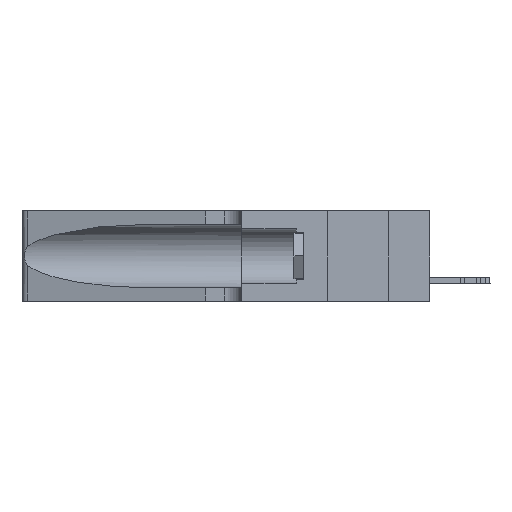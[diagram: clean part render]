
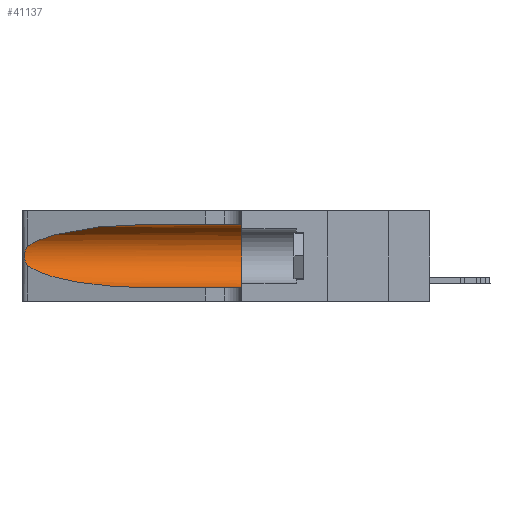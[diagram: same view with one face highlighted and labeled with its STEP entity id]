
A CAD part, left-side view. The second image highlights one B-rep face of the part: STEP entity #41137.
In plain terms, the highlighted cylindrical face has radius 3.308 mm (diameter 6.617 mm), a partial arc.
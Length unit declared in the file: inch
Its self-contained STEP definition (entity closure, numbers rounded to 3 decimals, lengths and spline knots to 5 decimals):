
#119 = CARTESIAN_POINT ( 'NONE',  ( 0.18966, 0.96281, 0.31525 ) ) ;
#580 = CARTESIAN_POINT ( 'NONE',  ( 0.26075, 1.23896, 0.178 ) ) ;
#2409 = B_SPLINE_CURVE_WITH_KNOTS ( 'NONE', 3,
 ( #41883, #7510, #21399, #31585, #34873, #38755, #18142, #580, #25042, #31433, #24588, #38159, #35306, #28150 ),
 .UNSPECIFIED., .F., .F.,
 ( 4, 2, 2, 2, 2, 2, 4 ),
 ( 0., 0.00027, 0.00053, 0.00107, 0.0016, 0.00187, 0.00214 ),
 .UNSPECIFIED. ) ;
#3069 = DIRECTION ( 'NONE',  ( 0., 0., -1. ) ) ;
#3190 = EDGE_CURVE ( 'NONE', #4982, #40101, #2409, .T. ) ;
#4982 = VERTEX_POINT ( 'NONE', #12054 ) ;
#5468 = EDGE_LOOP ( 'NONE', ( #38649, #18389, #15389, #16194, #5944, #16312 ) ) ;
#5537 = DIRECTION ( 'NONE',  ( 0., 1., 0. ) ) ;
#5944 = ORIENTED_EDGE ( 'NONE', *, *, #43632, .F. ) ;
#6344 = DIRECTION ( 'NONE',  ( 0., -1., 0. ) ) ;
#7048 = CARTESIAN_POINT ( 'NONE',  ( 0.25487, 1.22718, 0.22369 ) ) ;
#7213 = LINE ( 'NONE', #14071, #25946 ) ;
#7510 = CARTESIAN_POINT ( 'NONE',  ( 0.25555, 1.22994, 0.2215 ) ) ;
#9076 = CARTESIAN_POINT ( 'NONE',  ( 0.25487, 1.22718, 0.14631 ) ) ;
#11506 = CARTESIAN_POINT ( 'NONE',  ( 0.2373, 1.15595, 0.08982 ) ) ;
#11791 =( BOUNDED_CURVE ( )  B_SPLINE_CURVE ( 3, ( #34417, #119, #21623, #7048 ),
 .UNSPECIFIED., .F., .F. ) 
 B_SPLINE_CURVE_WITH_KNOTS ( ( 4, 4 ),
 ( 1.5708, 2.84003 ),
 .UNSPECIFIED. ) 
 CURVE ( )  GEOMETRIC_REPRESENTATION_ITEM ( )  RATIONAL_B_SPLINE_CURVE ( ( 1., 0.87, 0.87, 1. ) ) 
 REPRESENTATION_ITEM ( '' )  );
#12054 = CARTESIAN_POINT ( 'NONE',  ( 0.25487, 1.22718, 0.22369 ) ) ;
#12594 = CARTESIAN_POINT ( 'NONE',  ( 0.1305, 0.72297, 0.05475 ) ) ;
#13159 =( BOUNDED_CURVE ( )  B_SPLINE_CURVE ( 3, ( #18953, #11506, #25413, #15234 ),
 .UNSPECIFIED., .F., .T. ) 
 B_SPLINE_CURVE_WITH_KNOTS ( ( 4, 4 ),
 ( 3.44316, 4.71239 ),
 .UNSPECIFIED. ) 
 CURVE ( )  GEOMETRIC_REPRESENTATION_ITEM ( )  RATIONAL_B_SPLINE_CURVE ( ( 1., 0.87, 0.87, 1. ) ) 
 REPRESENTATION_ITEM ( '' )  );
#13620 = VERTEX_POINT ( 'NONE', #41635 ) ;
#14071 = CARTESIAN_POINT ( 'NONE',  ( 0.1305, 1.61858, 0.05475 ) ) ;
#15234 = CARTESIAN_POINT ( 'NONE',  ( 0.1305, 0.72297, 0.05475 ) ) ;
#15389 = ORIENTED_EDGE ( 'NONE', *, *, #36795, .T. ) ;
#16194 = ORIENTED_EDGE ( 'NONE', *, *, #42758, .T. ) ;
#16312 = ORIENTED_EDGE ( 'NONE', *, *, #21706, .F. ) ;
#16372 = VERTEX_POINT ( 'NONE', #29715 ) ;
#17800 = DIRECTION ( 'NONE',  ( 0., -1., 0. ) ) ;
#18142 = CARTESIAN_POINT ( 'NONE',  ( 0.26075, 1.23896, 0.19203 ) ) ;
#18389 = ORIENTED_EDGE ( 'NONE', *, *, #3190, .T. ) ;
#18699 = AXIS2_PLACEMENT_3D ( 'NONE', #32925, #5537, #18898 ) ;
#18898 = DIRECTION ( 'NONE',  ( 0., 0., 1. ) ) ;
#18953 = CARTESIAN_POINT ( 'NONE',  ( 0.25487, 1.22718, 0.14631 ) ) ;
#21399 = CARTESIAN_POINT ( 'NONE',  ( 0.25639, 1.23184, 0.21858 ) ) ;
#21623 = CARTESIAN_POINT ( 'NONE',  ( 0.2373, 1.15595, 0.28018 ) ) ;
#21706 = EDGE_CURVE ( 'NONE', #16372, #13620, #22456, .T. ) ;
#22456 = LINE ( 'NONE', #34005, #28370 ) ;
#23641 = VERTEX_POINT ( 'NONE', #12594 ) ;
#24464 = CIRCLE ( 'NONE', #18699, 0.13025 ) ;
#24588 = CARTESIAN_POINT ( 'NONE',  ( 0.25789, 1.23486, 0.15765 ) ) ;
#25042 = CARTESIAN_POINT ( 'NONE',  ( 0.26017, 1.23833, 0.17102 ) ) ;
#25413 = CARTESIAN_POINT ( 'NONE',  ( 0.18966, 0.96281, 0.05475 ) ) ;
#25946 = VECTOR ( 'NONE', #17800, 39.37008 ) ;
#26310 = EDGE_CURVE ( 'NONE', #16372, #4982, #11791, .T. ) ;
#27505 = VERTEX_POINT ( 'NONE', #28195 ) ;
#28150 = CARTESIAN_POINT ( 'NONE',  ( 0.25487, 1.22718, 0.14631 ) ) ;
#28195 = CARTESIAN_POINT ( 'NONE',  ( 0.1305, 0.35, 0.05475 ) ) ;
#28370 = VECTOR ( 'NONE', #6344, 39.37008 ) ;
#29715 = CARTESIAN_POINT ( 'NONE',  ( 0.1305, 0.72297, 0.31525 ) ) ;
#30481 = DIRECTION ( 'NONE',  ( 0., -1., 0. ) ) ;
#31433 = CARTESIAN_POINT ( 'NONE',  ( 0.25856, 1.23593, 0.16098 ) ) ;
#31585 = CARTESIAN_POINT ( 'NONE',  ( 0.25787, 1.23484, 0.2124 ) ) ;
#32925 = CARTESIAN_POINT ( 'NONE',  ( 0.1305, 0.35, 0.185 ) ) ;
#34005 = CARTESIAN_POINT ( 'NONE',  ( 0.1305, 1.61858, 0.31525 ) ) ;
#34082 = AXIS2_PLACEMENT_3D ( 'NONE', #36939, #30481, #3069 ) ;
#34417 = CARTESIAN_POINT ( 'NONE',  ( 0.1305, 0.72297, 0.31525 ) ) ;
#34677 = CYLINDRICAL_SURFACE ( 'NONE', #34082, 0.13025 ) ;
#34873 = CARTESIAN_POINT ( 'NONE',  ( 0.25854, 1.2359, 0.20912 ) ) ;
#35306 = CARTESIAN_POINT ( 'NONE',  ( 0.25555, 1.22993, 0.14849 ) ) ;
#36795 = EDGE_CURVE ( 'NONE', #40101, #23641, #13159, .T. ) ;
#36939 = CARTESIAN_POINT ( 'NONE',  ( 0.1305, 1.61858, 0.185 ) ) ;
#38159 = CARTESIAN_POINT ( 'NONE',  ( 0.25639, 1.23186, 0.15144 ) ) ;
#38649 = ORIENTED_EDGE ( 'NONE', *, *, #26310, .T. ) ;
#38755 = CARTESIAN_POINT ( 'NONE',  ( 0.26018, 1.23835, 0.19895 ) ) ;
#40101 = VERTEX_POINT ( 'NONE', #9076 ) ;
#41137 = ADVANCED_FACE ( 'NONE', ( #42670 ), #34677, .F. ) ;
#41635 = CARTESIAN_POINT ( 'NONE',  ( 0.1305, 0.35, 0.31525 ) ) ;
#41883 = CARTESIAN_POINT ( 'NONE',  ( 0.25487, 1.22718, 0.22369 ) ) ;
#42670 = FACE_OUTER_BOUND ( 'NONE', #5468, .T. ) ;
#42758 = EDGE_CURVE ( 'NONE', #23641, #27505, #7213, .T. ) ;
#43632 = EDGE_CURVE ( 'NONE', #13620, #27505, #24464, .T. ) ;
